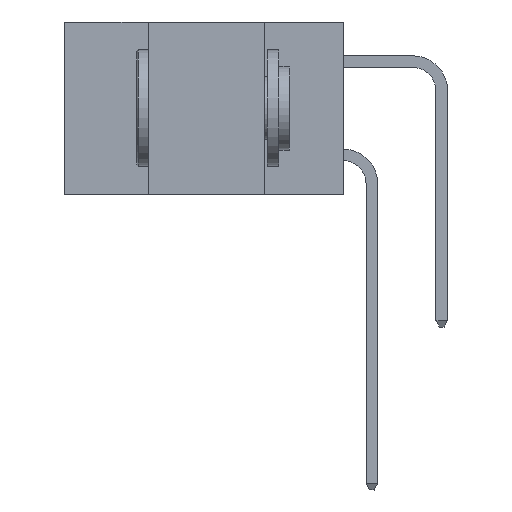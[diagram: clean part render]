
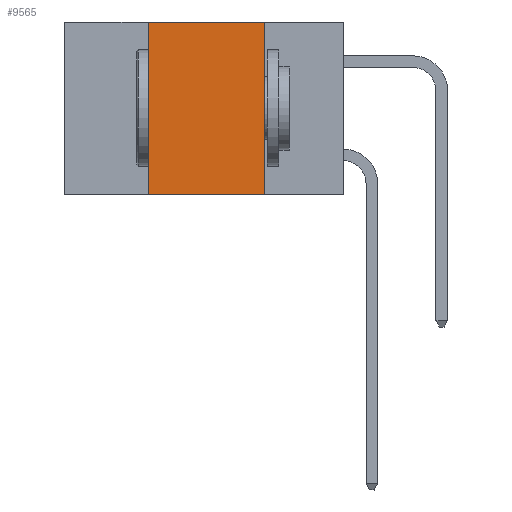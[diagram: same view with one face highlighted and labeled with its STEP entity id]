
A CAD part, left-side view. The second image highlights one B-rep face of the part: STEP entity #9565.
In plain terms, the highlighted planar face has unit normal (-1, 0, 0).
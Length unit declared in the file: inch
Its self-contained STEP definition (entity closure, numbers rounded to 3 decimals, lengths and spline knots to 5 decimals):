
#1035 = EDGE_CURVE ( 'NONE', #11601, #2068, #11866, .T. ) ;
#1247 = EDGE_CURVE ( 'NONE', #8846, #11601, #5993, .T. ) ;
#2068 = VERTEX_POINT ( 'NONE', #22485 ) ;
#2076 = CARTESIAN_POINT ( 'NONE',  ( 0., 0.6, 0. ) ) ;
#2085 = ORIENTED_EDGE ( 'NONE', *, *, #1035, .F. ) ;
#2432 = ORIENTED_EDGE ( 'NONE', *, *, #19977, .T. ) ;
#5993 = LINE ( 'NONE', #18111, #6710 ) ;
#6444 = DIRECTION ( 'NONE',  ( 0., 0., 1. ) ) ;
#6710 = VECTOR ( 'NONE', #6444, 39.37008 ) ;
#7877 = VECTOR ( 'NONE', #16737, 39.37008 ) ;
#8250 = FACE_OUTER_BOUND ( 'NONE', #19071, .T. ) ;
#8846 = VERTEX_POINT ( 'NONE', #24090 ) ;
#9376 = ORIENTED_EDGE ( 'NONE', *, *, #28345, .F. ) ;
#9565 = ADVANCED_FACE ( 'NONE', ( #8250 ), #27522, .F. ) ;
#9767 = VECTOR ( 'NONE', #23327, 39.37008 ) ;
#11601 = VERTEX_POINT ( 'NONE', #27304 ) ;
#11866 = LINE ( 'NONE', #28704, #23388 ) ;
#12066 = CARTESIAN_POINT ( 'NONE',  ( 0., 0.17, 0. ) ) ;
#16737 = DIRECTION ( 'NONE',  ( 0., -1., 0. ) ) ;
#17746 = AXIS2_PLACEMENT_3D ( 'NONE', #2076, #29967, #18277 ) ;
#18111 = CARTESIAN_POINT ( 'NONE',  ( 0., 0.42, 0. ) ) ;
#18277 = DIRECTION ( 'NONE',  ( 0., 0., -1. ) ) ;
#19071 = EDGE_LOOP ( 'NONE', ( #9376, #2085, #22281, #2432 ) ) ;
#19249 = CARTESIAN_POINT ( 'NONE',  ( 0., 0.6, -0.37 ) ) ;
#19977 = EDGE_CURVE ( 'NONE', #8846, #29144, #26291, .T. ) ;
#22226 = DIRECTION ( 'NONE',  ( 0., -1., 0. ) ) ;
#22281 = ORIENTED_EDGE ( 'NONE', *, *, #1247, .F. ) ;
#22485 = CARTESIAN_POINT ( 'NONE',  ( 0., 0.17, 0. ) ) ;
#22545 = CARTESIAN_POINT ( 'NONE',  ( 0., 0.17, -0.37 ) ) ;
#23327 = DIRECTION ( 'NONE',  ( 0., 0., -1. ) ) ;
#23388 = VECTOR ( 'NONE', #22226, 39.37008 ) ;
#24090 = CARTESIAN_POINT ( 'NONE',  ( 0., 0.42, -0.37 ) ) ;
#25263 = LINE ( 'NONE', #12066, #9767 ) ;
#26291 = LINE ( 'NONE', #19249, #7877 ) ;
#27304 = CARTESIAN_POINT ( 'NONE',  ( 0., 0.42, 0. ) ) ;
#27522 = PLANE ( 'NONE',  #17746 ) ;
#28345 = EDGE_CURVE ( 'NONE', #2068, #29144, #25263, .T. ) ;
#28704 = CARTESIAN_POINT ( 'NONE',  ( 0., 0.6, 0. ) ) ;
#29144 = VERTEX_POINT ( 'NONE', #22545 ) ;
#29967 = DIRECTION ( 'NONE',  ( 1., 0., 0. ) ) ;
